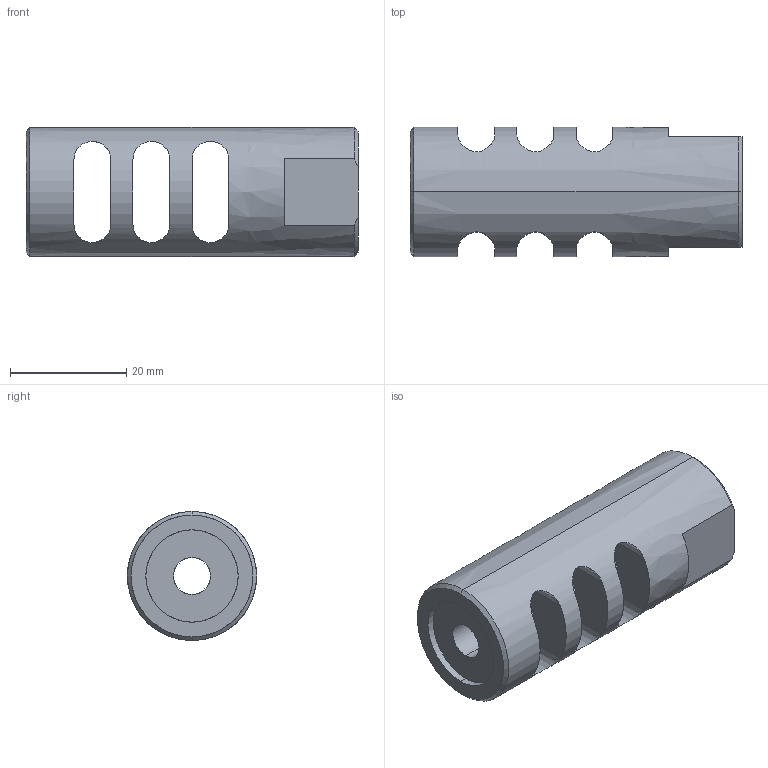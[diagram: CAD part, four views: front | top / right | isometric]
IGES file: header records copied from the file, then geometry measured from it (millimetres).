
Start section: SolidWorks IGES file using analytic representation for surfaces
Global section: file name: Muzzle Break.IGS; native system: SolidWorks 2011; preprocessor: SolidWorks 2011; author: Shane; date: 120428.221937; units: inch
Bounding box: 57.15 x 22.23 x 22.23 mm (x, y, z)
Surface area: 7200.8 mm2 (no closed solid volume)
Topology: 0 solids, 0 shells, 42 faces, 1111 edges, 1111 vertices
Faces by surface type: revolution 28, bspline 14
